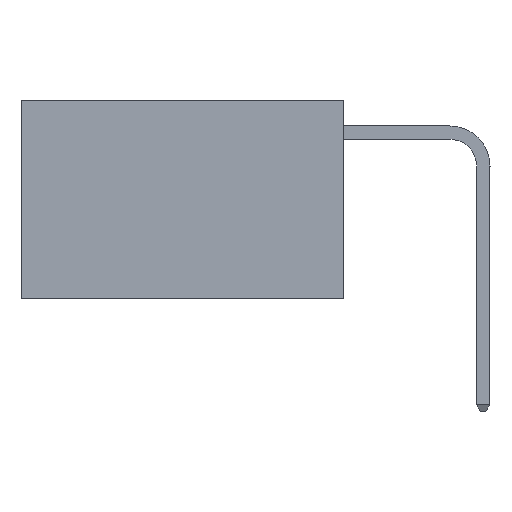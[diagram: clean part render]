
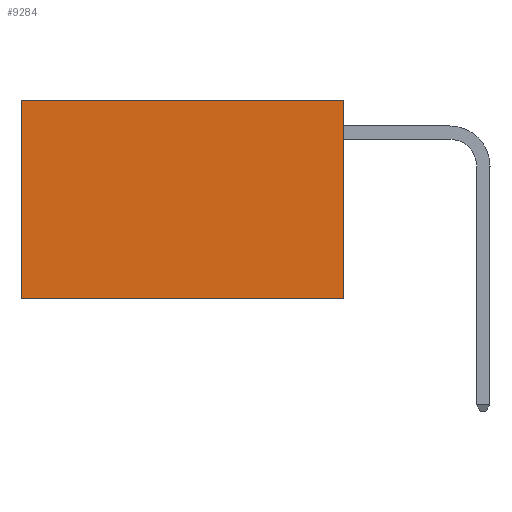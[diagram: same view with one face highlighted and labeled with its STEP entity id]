
A CAD part, left-side view. The second image highlights one B-rep face of the part: STEP entity #9284.
In plain terms, the highlighted planar face has unit normal (-1, 0, 0).
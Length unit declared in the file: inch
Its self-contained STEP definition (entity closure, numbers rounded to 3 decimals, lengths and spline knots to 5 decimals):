
#6 = LINE ( 'NONE', #8032, #3048 ) ;
#104 = DIRECTION ( 'NONE',  ( 0., 1., 0. ) ) ;
#652 = CARTESIAN_POINT ( 'NONE',  ( 0.2625, 0., 0. ) ) ;
#885 = DIRECTION ( 'NONE',  ( 0., 0., -1. ) ) ;
#1524 = VERTEX_POINT ( 'NONE', #10049 ) ;
#1638 = DIRECTION ( 'NONE',  ( 0., 0., -1. ) ) ;
#1763 = VECTOR ( 'NONE', #104, 39.37008 ) ;
#1823 = DIRECTION ( 'NONE',  ( 0., 0., -1. ) ) ;
#2115 = LINE ( 'NONE', #2364, #1763 ) ;
#2130 = ORIENTED_EDGE ( 'NONE', *, *, #13536, .F. ) ;
#2224 = AXIS2_PLACEMENT_3D ( 'NONE', #652, #8209, #1823 ) ;
#2364 = CARTESIAN_POINT ( 'NONE',  ( 0.2625, 0., 0. ) ) ;
#2473 = ORIENTED_EDGE ( 'NONE', *, *, #8939, .T. ) ;
#2564 = VERTEX_POINT ( 'NONE', #9808 ) ;
#2812 = FACE_OUTER_BOUND ( 'NONE', #13109, .T. ) ;
#3048 = VECTOR ( 'NONE', #1638, 39.37008 ) ;
#3222 = VECTOR ( 'NONE', #885, 39.37008 ) ;
#4884 = CARTESIAN_POINT ( 'NONE',  ( 0.2625, 0., -0.37 ) ) ;
#4975 = ORIENTED_EDGE ( 'NONE', *, *, #11008, .F. ) ;
#5726 = LINE ( 'NONE', #4884, #11010 ) ;
#6063 = PLANE ( 'NONE',  #2224 ) ;
#6768 = ORIENTED_EDGE ( 'NONE', *, *, #13248, .T. ) ;
#8032 = CARTESIAN_POINT ( 'NONE',  ( 0.2625, 0.6, 0. ) ) ;
#8073 = VERTEX_POINT ( 'NONE', #13500 ) ;
#8209 = DIRECTION ( 'NONE',  ( 1., 0., 0. ) ) ;
#8479 = LINE ( 'NONE', #11527, #3222 ) ;
#8643 = CARTESIAN_POINT ( 'NONE',  ( 0.2625, 0.6, 0. ) ) ;
#8939 = EDGE_CURVE ( 'NONE', #8073, #10686, #2115, .T. ) ;
#9284 = ADVANCED_FACE ( 'NONE', ( #2812 ), #6063, .F. ) ;
#9808 = CARTESIAN_POINT ( 'NONE',  ( 0.2625, 0., -0.37 ) ) ;
#10049 = CARTESIAN_POINT ( 'NONE',  ( 0.2625, 0.6, -0.37 ) ) ;
#10686 = VERTEX_POINT ( 'NONE', #8643 ) ;
#11008 = EDGE_CURVE ( 'NONE', #2564, #1524, #5726, .T. ) ;
#11010 = VECTOR ( 'NONE', #11208, 39.37008 ) ;
#11208 = DIRECTION ( 'NONE',  ( 0., 1., 0. ) ) ;
#11527 = CARTESIAN_POINT ( 'NONE',  ( 0.2625, 0., 0. ) ) ;
#13109 = EDGE_LOOP ( 'NONE', ( #6768, #4975, #2130, #2473 ) ) ;
#13248 = EDGE_CURVE ( 'NONE', #10686, #1524, #6, .T. ) ;
#13500 = CARTESIAN_POINT ( 'NONE',  ( 0.2625, 0., 0. ) ) ;
#13536 = EDGE_CURVE ( 'NONE', #8073, #2564, #8479, .T. ) ;
